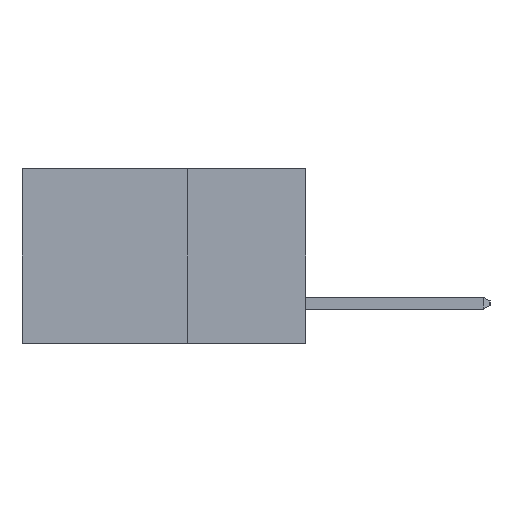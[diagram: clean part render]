
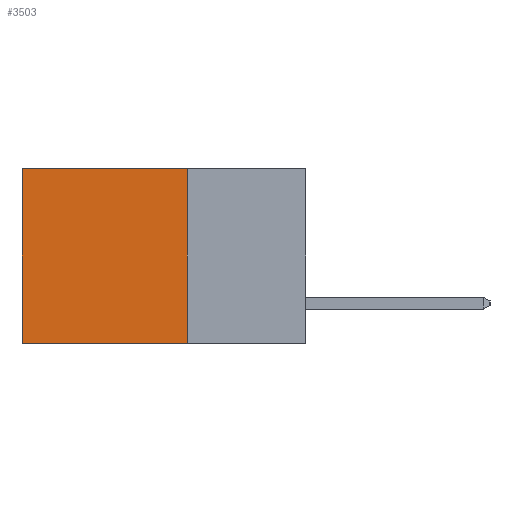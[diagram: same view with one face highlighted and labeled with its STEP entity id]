
A CAD part, left-side view. The second image highlights one B-rep face of the part: STEP entity #3503.
In plain terms, the highlighted planar face has unit normal (-1, 0, 0).
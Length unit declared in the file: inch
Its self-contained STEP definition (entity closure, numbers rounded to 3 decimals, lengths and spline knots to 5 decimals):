
#19 = AXIS2_PLACEMENT_3D ( 'NONE', #2035, #4356, #4386 ) ;
#51 = DIRECTION ( 'NONE',  ( 0., 1., 0. ) ) ;
#284 = VERTEX_POINT ( 'NONE', #4066 ) ;
#398 = ORIENTED_EDGE ( 'NONE', *, *, #5430, .T. ) ;
#805 = VECTOR ( 'NONE', #7878, 39.37008 ) ;
#839 = PLANE ( 'NONE',  #19 ) ;
#1083 = CARTESIAN_POINT ( 'NONE',  ( 0.298, 0.6, -0.37 ) ) ;
#1096 = LINE ( 'NONE', #6964, #805 ) ;
#1108 = VECTOR ( 'NONE', #51, 39.37008 ) ;
#1159 = ORIENTED_EDGE ( 'NONE', *, *, #5553, .F. ) ;
#1401 = LINE ( 'NONE', #8982, #1108 ) ;
#2035 = CARTESIAN_POINT ( 'NONE',  ( 0.298, 0.25, 0. ) ) ;
#2094 = LINE ( 'NONE', #8899, #11182 ) ;
#2743 = EDGE_LOOP ( 'NONE', ( #10503, #5269, #1159, #398 ) ) ;
#3503 = ADVANCED_FACE ( 'NONE', ( #10112 ), #839, .F. ) ;
#3595 = CARTESIAN_POINT ( 'NONE',  ( 0.298, 0.6, 0. ) ) ;
#3620 = VERTEX_POINT ( 'NONE', #8796 ) ;
#3657 = CARTESIAN_POINT ( 'NONE',  ( 0.298, 0.6, 0. ) ) ;
#4066 = CARTESIAN_POINT ( 'NONE',  ( 0.298, 0.25, -0.37 ) ) ;
#4356 = DIRECTION ( 'NONE',  ( 1., 0., 0. ) ) ;
#4386 = DIRECTION ( 'NONE',  ( 0., 0., -1. ) ) ;
#4994 = EDGE_CURVE ( 'NONE', #284, #8493, #1401, .T. ) ;
#5269 = ORIENTED_EDGE ( 'NONE', *, *, #4994, .F. ) ;
#5394 = DIRECTION ( 'NONE',  ( 0., 0., -1. ) ) ;
#5430 = EDGE_CURVE ( 'NONE', #3620, #5500, #1096, .T. ) ;
#5500 = VERTEX_POINT ( 'NONE', #3595 ) ;
#5553 = EDGE_CURVE ( 'NONE', #3620, #284, #2094, .T. ) ;
#5993 = VECTOR ( 'NONE', #8884, 39.37008 ) ;
#6160 = EDGE_CURVE ( 'NONE', #5500, #8493, #10686, .T. ) ;
#6964 = CARTESIAN_POINT ( 'NONE',  ( 0.298, 0.25, 0. ) ) ;
#7878 = DIRECTION ( 'NONE',  ( 0., 1., 0. ) ) ;
#8493 = VERTEX_POINT ( 'NONE', #1083 ) ;
#8796 = CARTESIAN_POINT ( 'NONE',  ( 0.298, 0.25, 0. ) ) ;
#8884 = DIRECTION ( 'NONE',  ( 0., 0., -1. ) ) ;
#8899 = CARTESIAN_POINT ( 'NONE',  ( 0.298, 0.25, 0. ) ) ;
#8982 = CARTESIAN_POINT ( 'NONE',  ( 0.298, 0.25, -0.37 ) ) ;
#10112 = FACE_OUTER_BOUND ( 'NONE', #2743, .T. ) ;
#10503 = ORIENTED_EDGE ( 'NONE', *, *, #6160, .T. ) ;
#10686 = LINE ( 'NONE', #3657, #5993 ) ;
#11182 = VECTOR ( 'NONE', #5394, 39.37008 ) ;
